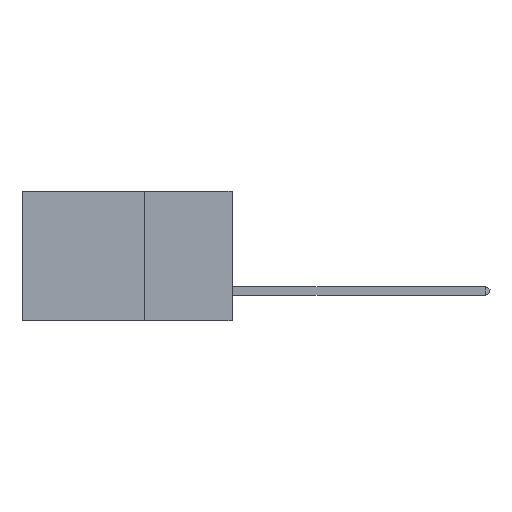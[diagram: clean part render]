
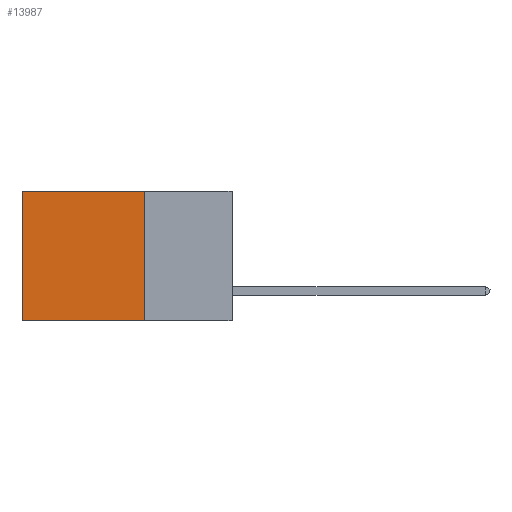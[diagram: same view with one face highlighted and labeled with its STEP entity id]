
A CAD part, left-side view. The second image highlights one B-rep face of the part: STEP entity #13987.
In plain terms, the highlighted planar face has unit normal (-1, 0, 0).
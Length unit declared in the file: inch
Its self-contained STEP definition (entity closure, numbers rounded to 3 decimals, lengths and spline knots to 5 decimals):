
#6 = DIRECTION ( 'NONE',  ( 1., 0., 0. ) ) ;
#861 = CARTESIAN_POINT ( 'NONE',  ( 0.2875, 0.25, -0.37 ) ) ;
#953 = LINE ( 'NONE', #6198, #9196 ) ;
#1524 = CARTESIAN_POINT ( 'NONE',  ( 0.2875, 0.6, 0. ) ) ;
#1916 = ORIENTED_EDGE ( 'NONE', *, *, #11187, .F. ) ;
#1952 = CARTESIAN_POINT ( 'NONE',  ( 0.2875, 0.6, -0.37 ) ) ;
#2036 = VERTEX_POINT ( 'NONE', #8893 ) ;
#3574 = VECTOR ( 'NONE', #8399, 39.37008 ) ;
#3776 = DIRECTION ( 'NONE',  ( 0., 0., -1. ) ) ;
#3829 = PLANE ( 'NONE',  #14935 ) ;
#3870 = EDGE_CURVE ( 'NONE', #2036, #14129, #4381, .T. ) ;
#4101 = CARTESIAN_POINT ( 'NONE',  ( 0.2875, 0.6, 0. ) ) ;
#4305 = LINE ( 'NONE', #4101, #5097 ) ;
#4381 = LINE ( 'NONE', #9804, #3574 ) ;
#5097 = VECTOR ( 'NONE', #12676, 39.37008 ) ;
#6198 = CARTESIAN_POINT ( 'NONE',  ( 0.2875, 0.25, 0. ) ) ;
#7472 = ORIENTED_EDGE ( 'NONE', *, *, #13962, .F. ) ;
#7825 = CARTESIAN_POINT ( 'NONE',  ( 0.2875, 0.25, -0.37 ) ) ;
#8380 = VECTOR ( 'NONE', #10382, 39.37008 ) ;
#8399 = DIRECTION ( 'NONE',  ( 0., 1., 0. ) ) ;
#8520 = VERTEX_POINT ( 'NONE', #861 ) ;
#8893 = CARTESIAN_POINT ( 'NONE',  ( 0.2875, 0.25, 0. ) ) ;
#8990 = FACE_OUTER_BOUND ( 'NONE', #13086, .T. ) ;
#9073 = ORIENTED_EDGE ( 'NONE', *, *, #3870, .T. ) ;
#9196 = VECTOR ( 'NONE', #9938, 39.37008 ) ;
#9804 = CARTESIAN_POINT ( 'NONE',  ( 0.2875, 0.25, 0. ) ) ;
#9933 = LINE ( 'NONE', #7825, #8380 ) ;
#9938 = DIRECTION ( 'NONE',  ( 0., 0., -1. ) ) ;
#10128 = ORIENTED_EDGE ( 'NONE', *, *, #14063, .T. ) ;
#10382 = DIRECTION ( 'NONE',  ( 0., 1., 0. ) ) ;
#10915 = VERTEX_POINT ( 'NONE', #1952 ) ;
#11187 = EDGE_CURVE ( 'NONE', #8520, #10915, #9933, .T. ) ;
#12676 = DIRECTION ( 'NONE',  ( 0., 0., -1. ) ) ;
#13086 = EDGE_LOOP ( 'NONE', ( #10128, #1916, #7472, #9073 ) ) ;
#13962 = EDGE_CURVE ( 'NONE', #2036, #8520, #953, .T. ) ;
#13987 = ADVANCED_FACE ( 'NONE', ( #8990 ), #3829, .F. ) ;
#14063 = EDGE_CURVE ( 'NONE', #14129, #10915, #4305, .T. ) ;
#14129 = VERTEX_POINT ( 'NONE', #1524 ) ;
#14929 = CARTESIAN_POINT ( 'NONE',  ( 0.2875, 0.25, 0. ) ) ;
#14935 = AXIS2_PLACEMENT_3D ( 'NONE', #14929, #6, #3776 ) ;
